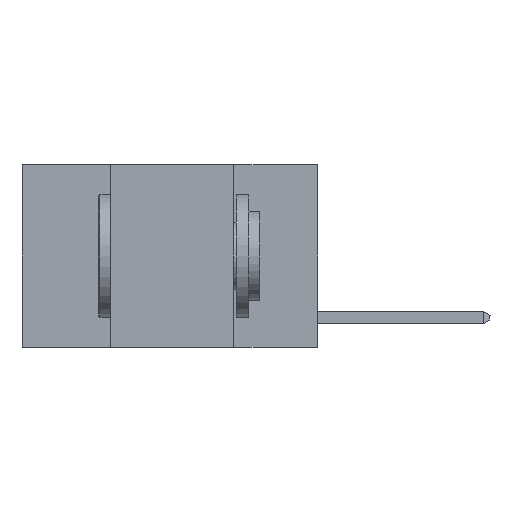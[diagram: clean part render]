
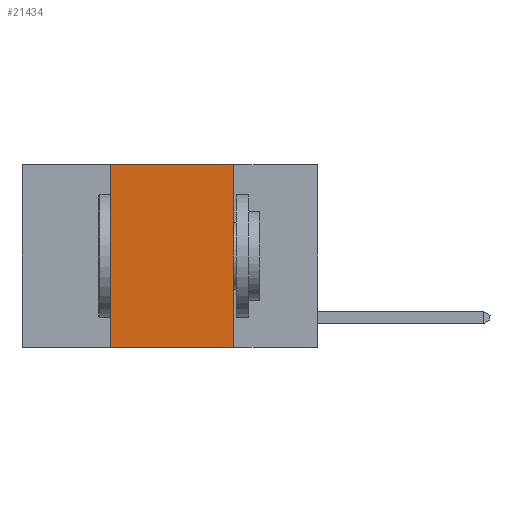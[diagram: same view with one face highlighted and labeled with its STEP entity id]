
A CAD part, left-side view. The second image highlights one B-rep face of the part: STEP entity #21434.
In plain terms, the highlighted planar face has unit normal (-1, 0, 0).
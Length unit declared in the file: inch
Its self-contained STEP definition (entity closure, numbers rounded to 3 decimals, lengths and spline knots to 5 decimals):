
#743 = VECTOR ( 'NONE', #7169, 39.37008 ) ;
#1820 = VECTOR ( 'NONE', #15681, 39.37008 ) ;
#2518 = LINE ( 'NONE', #4530, #743 ) ;
#2940 = EDGE_LOOP ( 'NONE', ( #5095, #21231, #3857, #22736 ) ) ;
#3857 = ORIENTED_EDGE ( 'NONE', *, *, #24101, .F. ) ;
#3893 = EDGE_CURVE ( 'NONE', #8436, #15887, #24446, .T. ) ;
#4530 = CARTESIAN_POINT ( 'NONE',  ( 0., 0.42, 0. ) ) ;
#5095 = ORIENTED_EDGE ( 'NONE', *, *, #18313, .F. ) ;
#6511 = DIRECTION ( 'NONE',  ( 0., -1., 0. ) ) ;
#6663 = DIRECTION ( 'NONE',  ( 0., 0., -1. ) ) ;
#7169 = DIRECTION ( 'NONE',  ( 0., 0., 1. ) ) ;
#8436 = VERTEX_POINT ( 'NONE', #8772 ) ;
#8504 = PLANE ( 'NONE',  #21564 ) ;
#8772 = CARTESIAN_POINT ( 'NONE',  ( 0., 0.42, 0. ) ) ;
#10253 = FACE_OUTER_BOUND ( 'NONE', #2940, .T. ) ;
#10460 = CARTESIAN_POINT ( 'NONE',  ( 0., 0.6, -0.37 ) ) ;
#12619 = DIRECTION ( 'NONE',  ( 0., -1., 0. ) ) ;
#13410 = CARTESIAN_POINT ( 'NONE',  ( 0., 0.17, -0.37 ) ) ;
#13626 = VECTOR ( 'NONE', #6511, 39.37008 ) ;
#13812 = LINE ( 'NONE', #15926, #1820 ) ;
#15681 = DIRECTION ( 'NONE',  ( 0., 0., -1. ) ) ;
#15887 = VERTEX_POINT ( 'NONE', #20777 ) ;
#15926 = CARTESIAN_POINT ( 'NONE',  ( 0., 0.17, 0. ) ) ;
#16023 = LINE ( 'NONE', #10460, #13626 ) ;
#17452 = VERTEX_POINT ( 'NONE', #13410 ) ;
#17958 = CARTESIAN_POINT ( 'NONE',  ( 0., 0.6, 0. ) ) ;
#18313 = EDGE_CURVE ( 'NONE', #15887, #17452, #13812, .T. ) ;
#19324 = CARTESIAN_POINT ( 'NONE',  ( 0., 0.42, -0.37 ) ) ;
#20203 = VECTOR ( 'NONE', #12619, 39.37008 ) ;
#20777 = CARTESIAN_POINT ( 'NONE',  ( 0., 0.17, 0. ) ) ;
#21231 = ORIENTED_EDGE ( 'NONE', *, *, #3893, .F. ) ;
#21434 = ADVANCED_FACE ( 'NONE', ( #10253 ), #8504, .F. ) ;
#21564 = AXIS2_PLACEMENT_3D ( 'NONE', #17958, #23621, #6663 ) ;
#22736 = ORIENTED_EDGE ( 'NONE', *, *, #23784, .T. ) ;
#23621 = DIRECTION ( 'NONE',  ( 1., 0., 0. ) ) ;
#23726 = VERTEX_POINT ( 'NONE', #19324 ) ;
#23784 = EDGE_CURVE ( 'NONE', #23726, #17452, #16023, .T. ) ;
#24101 = EDGE_CURVE ( 'NONE', #23726, #8436, #2518, .T. ) ;
#24446 = LINE ( 'NONE', #24714, #20203 ) ;
#24714 = CARTESIAN_POINT ( 'NONE',  ( 0., 0.6, 0. ) ) ;
